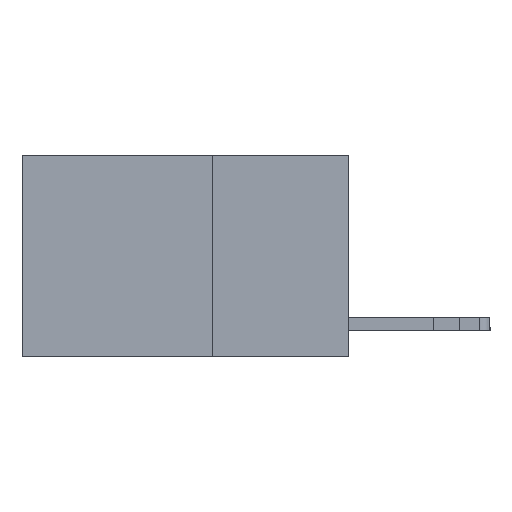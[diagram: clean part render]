
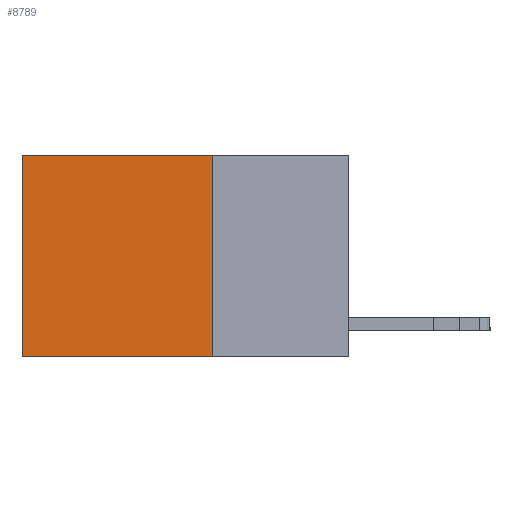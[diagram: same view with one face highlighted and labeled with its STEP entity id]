
A CAD part, left-side view. The second image highlights one B-rep face of the part: STEP entity #8789.
In plain terms, the highlighted planar face has unit normal (-1, 0, 0).
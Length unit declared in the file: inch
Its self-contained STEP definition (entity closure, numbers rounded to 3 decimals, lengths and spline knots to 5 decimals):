
#441 = ORIENTED_EDGE ( 'NONE', *, *, #1585, .T. ) ;
#685 = LINE ( 'NONE', #16003, #14142 ) ;
#1585 = EDGE_CURVE ( 'NONE', #18381, #3488, #685, .T. ) ;
#1923 = ORIENTED_EDGE ( 'NONE', *, *, #15613, .F. ) ;
#3488 = VERTEX_POINT ( 'NONE', #8300 ) ;
#3748 = CARTESIAN_POINT ( 'NONE',  ( 0.2625, 0.25, 0. ) ) ;
#3873 = DIRECTION ( 'NONE',  ( 0., 0., -1. ) ) ;
#4811 = PLANE ( 'NONE',  #16398 ) ;
#4832 = DIRECTION ( 'NONE',  ( 0., 1., 0. ) ) ;
#5453 = VECTOR ( 'NONE', #7825, 39.37008 ) ;
#6835 = DIRECTION ( 'NONE',  ( 0., 1., 0. ) ) ;
#7041 = CARTESIAN_POINT ( 'NONE',  ( 0.2625, 0.25, -0.37 ) ) ;
#7541 = DIRECTION ( 'NONE',  ( 0., 0., -1. ) ) ;
#7770 = CARTESIAN_POINT ( 'NONE',  ( 0.2625, 0.25, -0.37 ) ) ;
#7825 = DIRECTION ( 'NONE',  ( 0., 0., -1. ) ) ;
#7947 = CARTESIAN_POINT ( 'NONE',  ( 0.2625, 0.6, -0.37 ) ) ;
#8025 = CARTESIAN_POINT ( 'NONE',  ( 0.2625, 0.25, 0. ) ) ;
#8300 = CARTESIAN_POINT ( 'NONE',  ( 0.2625, 0.6, 0. ) ) ;
#8741 = VERTEX_POINT ( 'NONE', #7947 ) ;
#8789 = ADVANCED_FACE ( 'NONE', ( #11452 ), #4811, .F. ) ;
#8830 = VECTOR ( 'NONE', #7541, 39.37008 ) ;
#9069 = LINE ( 'NONE', #10466, #8830 ) ;
#9676 = EDGE_LOOP ( 'NONE', ( #10935, #1923, #10606, #441 ) ) ;
#9842 = DIRECTION ( 'NONE',  ( 1., 0., 0. ) ) ;
#10466 = CARTESIAN_POINT ( 'NONE',  ( 0.2625, 0.6, 0. ) ) ;
#10606 = ORIENTED_EDGE ( 'NONE', *, *, #13767, .F. ) ;
#10935 = ORIENTED_EDGE ( 'NONE', *, *, #15866, .T. ) ;
#10982 = CARTESIAN_POINT ( 'NONE',  ( 0.2625, 0.25, 0. ) ) ;
#11452 = FACE_OUTER_BOUND ( 'NONE', #9676, .T. ) ;
#11653 = VERTEX_POINT ( 'NONE', #7041 ) ;
#13767 = EDGE_CURVE ( 'NONE', #18381, #11653, #15681, .T. ) ;
#14142 = VECTOR ( 'NONE', #6835, 39.37008 ) ;
#15535 = LINE ( 'NONE', #7770, #19103 ) ;
#15613 = EDGE_CURVE ( 'NONE', #11653, #8741, #15535, .T. ) ;
#15681 = LINE ( 'NONE', #8025, #5453 ) ;
#15866 = EDGE_CURVE ( 'NONE', #3488, #8741, #9069, .T. ) ;
#16003 = CARTESIAN_POINT ( 'NONE',  ( 0.2625, 0.25, 0. ) ) ;
#16398 = AXIS2_PLACEMENT_3D ( 'NONE', #10982, #9842, #3873 ) ;
#18381 = VERTEX_POINT ( 'NONE', #3748 ) ;
#19103 = VECTOR ( 'NONE', #4832, 39.37008 ) ;
